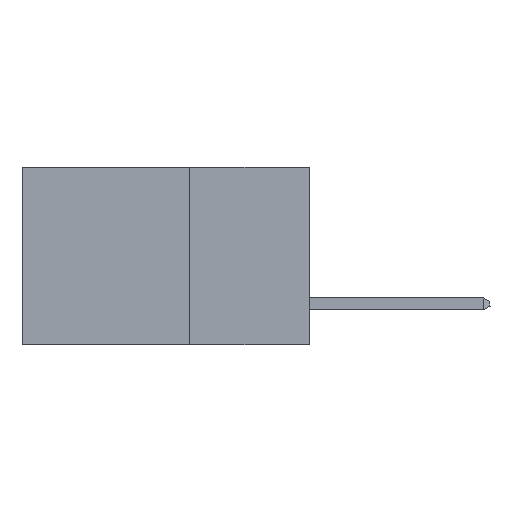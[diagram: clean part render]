
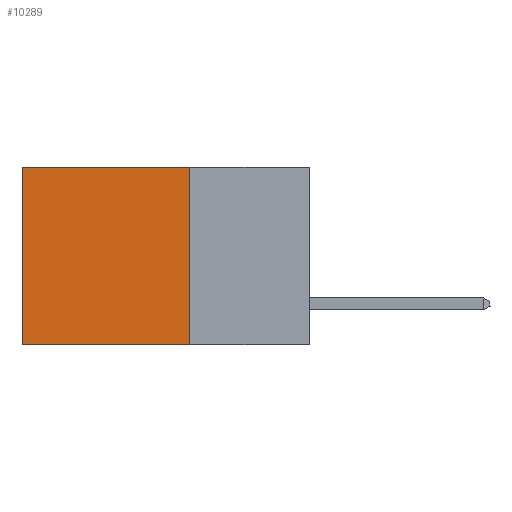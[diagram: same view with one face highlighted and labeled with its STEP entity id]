
A CAD part, left-side view. The second image highlights one B-rep face of the part: STEP entity #10289.
In plain terms, the highlighted planar face has unit normal (-1, 0, 0).
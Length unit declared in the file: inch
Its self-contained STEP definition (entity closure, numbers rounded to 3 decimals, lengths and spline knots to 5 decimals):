
#2260 = ORIENTED_EDGE ( 'NONE', *, *, #32464, .T. ) ;
#3541 = DIRECTION ( 'NONE',  ( 1., 0., 0. ) ) ;
#4504 = EDGE_CURVE ( 'NONE', #22807, #13799, #35160, .T. ) ;
#6778 = VERTEX_POINT ( 'NONE', #11192 ) ;
#7346 = EDGE_CURVE ( 'NONE', #6778, #13799, #42056, .T. ) ;
#7732 = AXIS2_PLACEMENT_3D ( 'NONE', #19859, #3541, #20425 ) ;
#9002 = CARTESIAN_POINT ( 'NONE',  ( 0.2875, 0.6, 0. ) ) ;
#10120 = DIRECTION ( 'NONE',  ( 0., 0., -1. ) ) ;
#10289 = ADVANCED_FACE ( 'NONE', ( #23604 ), #21340, .F. ) ;
#11192 = CARTESIAN_POINT ( 'NONE',  ( 0.2875, 0.6, 0. ) ) ;
#11719 = CARTESIAN_POINT ( 'NONE',  ( 0.2875, 0.6, -0.37 ) ) ;
#12630 = LINE ( 'NONE', #33500, #40137 ) ;
#13362 = CARTESIAN_POINT ( 'NONE',  ( 0.2875, 0.25, 0. ) ) ;
#13799 = VERTEX_POINT ( 'NONE', #11719 ) ;
#15151 = DIRECTION ( 'NONE',  ( 0., 1., 0. ) ) ;
#15526 = EDGE_LOOP ( 'NONE', ( #41498, #29700, #20712, #2260 ) ) ;
#17431 = DIRECTION ( 'NONE',  ( 0., 0., -1. ) ) ;
#19578 = VECTOR ( 'NONE', #33011, 39.37008 ) ;
#19859 = CARTESIAN_POINT ( 'NONE',  ( 0.2875, 0.25, 0. ) ) ;
#20425 = DIRECTION ( 'NONE',  ( 0., 0., -1. ) ) ;
#20712 = ORIENTED_EDGE ( 'NONE', *, *, #29473, .F. ) ;
#21077 = LINE ( 'NONE', #13362, #19578 ) ;
#21340 = PLANE ( 'NONE',  #7732 ) ;
#22807 = VERTEX_POINT ( 'NONE', #26772 ) ;
#23604 = FACE_OUTER_BOUND ( 'NONE', #15526, .T. ) ;
#25265 = CARTESIAN_POINT ( 'NONE',  ( 0.2875, 0.25, -0.37 ) ) ;
#25468 = VECTOR ( 'NONE', #15151, 39.37008 ) ;
#26772 = CARTESIAN_POINT ( 'NONE',  ( 0.2875, 0.25, -0.37 ) ) ;
#29473 = EDGE_CURVE ( 'NONE', #37762, #22807, #12630, .T. ) ;
#29700 = ORIENTED_EDGE ( 'NONE', *, *, #4504, .F. ) ;
#32464 = EDGE_CURVE ( 'NONE', #37762, #6778, #21077, .T. ) ;
#33011 = DIRECTION ( 'NONE',  ( 0., 1., 0. ) ) ;
#33396 = VECTOR ( 'NONE', #10120, 39.37008 ) ;
#33500 = CARTESIAN_POINT ( 'NONE',  ( 0.2875, 0.25, 0. ) ) ;
#35160 = LINE ( 'NONE', #25265, #25468 ) ;
#37762 = VERTEX_POINT ( 'NONE', #38220 ) ;
#38220 = CARTESIAN_POINT ( 'NONE',  ( 0.2875, 0.25, 0. ) ) ;
#40137 = VECTOR ( 'NONE', #17431, 39.37008 ) ;
#41498 = ORIENTED_EDGE ( 'NONE', *, *, #7346, .T. ) ;
#42056 = LINE ( 'NONE', #9002, #33396 ) ;
